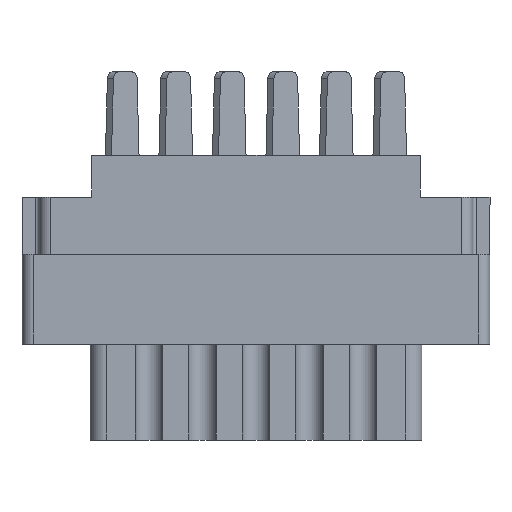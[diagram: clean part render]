
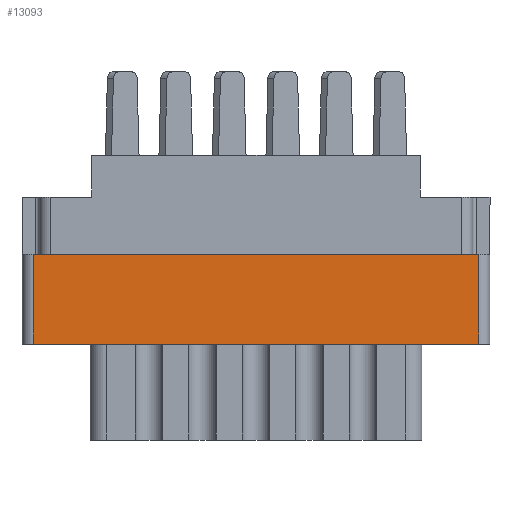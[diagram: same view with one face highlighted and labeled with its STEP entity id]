
A CAD part, front view. The second image highlights one B-rep face of the part: STEP entity #13093.
In plain terms, the highlighted planar face has unit normal (0, -1, 0).
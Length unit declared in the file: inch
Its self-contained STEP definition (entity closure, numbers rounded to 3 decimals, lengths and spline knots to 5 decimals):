
#209 = EDGE_CURVE ( 'NONE', #12823, #14746, #676, .T. ) ;
#676 = LINE ( 'NONE', #11794, #13753 ) ;
#979 = VERTEX_POINT ( 'NONE', #20664 ) ;
#1037 = VECTOR ( 'NONE', #12535, 39.37008 ) ;
#2098 = ORIENTED_EDGE ( 'NONE', *, *, #18703, .F. ) ;
#2555 = ORIENTED_EDGE ( 'NONE', *, *, #4022, .F. ) ;
#4022 = EDGE_CURVE ( 'NONE', #14746, #979, #20772, .T. ) ;
#4596 = DIRECTION ( 'NONE',  ( 1., 0., 0. ) ) ;
#5087 = VERTEX_POINT ( 'NONE', #5596 ) ;
#5596 = CARTESIAN_POINT ( 'NONE',  ( 0.624, -0.343, -0.277 ) ) ;
#5643 = ORIENTED_EDGE ( 'NONE', *, *, #10950, .T. ) ;
#6736 = CARTESIAN_POINT ( 'NONE',  ( -0.656, -0.343, -0.277 ) ) ;
#6741 = DIRECTION ( 'NONE',  ( 0., 0., -1. ) ) ;
#7969 = ORIENTED_EDGE ( 'NONE', *, *, #209, .F. ) ;
#9755 = DIRECTION ( 'NONE',  ( -1., 0., 0. ) ) ;
#9872 = CARTESIAN_POINT ( 'NONE',  ( -0.624, -0.343, -0.798 ) ) ;
#9893 = CARTESIAN_POINT ( 'NONE',  ( -0.624, -0.343, -0.798 ) ) ;
#10950 = EDGE_CURVE ( 'NONE', #12823, #5087, #16345, .T. ) ;
#11794 = CARTESIAN_POINT ( 'NONE',  ( 0.624, -0.343, -0.529 ) ) ;
#12535 = DIRECTION ( 'NONE',  ( 0., 0., 1. ) ) ;
#12653 = CARTESIAN_POINT ( 'NONE',  ( 0.624, -0.343, -0.798 ) ) ;
#12823 = VERTEX_POINT ( 'NONE', #14525 ) ;
#13093 = ADVANCED_FACE ( 'NONE', ( #20863 ), #21103, .T. ) ;
#13170 = EDGE_LOOP ( 'NONE', ( #2555, #7969, #5643, #2098 ) ) ;
#13592 = DIRECTION ( 'NONE',  ( 0., 0., 1. ) ) ;
#13753 = VECTOR ( 'NONE', #9755, 39.37008 ) ;
#14525 = CARTESIAN_POINT ( 'NONE',  ( 0.624, -0.343, -0.529 ) ) ;
#14746 = VERTEX_POINT ( 'NONE', #15466 ) ;
#15466 = CARTESIAN_POINT ( 'NONE',  ( -0.624, -0.343, -0.529 ) ) ;
#15499 = VECTOR ( 'NONE', #4596, 39.37008 ) ;
#15712 = LINE ( 'NONE', #6736, #15499 ) ;
#15735 = AXIS2_PLACEMENT_3D ( 'NONE', #9872, #17393, #6741 ) ;
#16345 = LINE ( 'NONE', #12653, #1037 ) ;
#17393 = DIRECTION ( 'NONE',  ( 0., -1., 0. ) ) ;
#18703 = EDGE_CURVE ( 'NONE', #979, #5087, #15712, .T. ) ;
#20664 = CARTESIAN_POINT ( 'NONE',  ( -0.624, -0.343, -0.277 ) ) ;
#20772 = LINE ( 'NONE', #9893, #20882 ) ;
#20863 = FACE_OUTER_BOUND ( 'NONE', #13170, .T. ) ;
#20882 = VECTOR ( 'NONE', #13592, 39.37008 ) ;
#21103 = PLANE ( 'NONE',  #15735 ) ;
